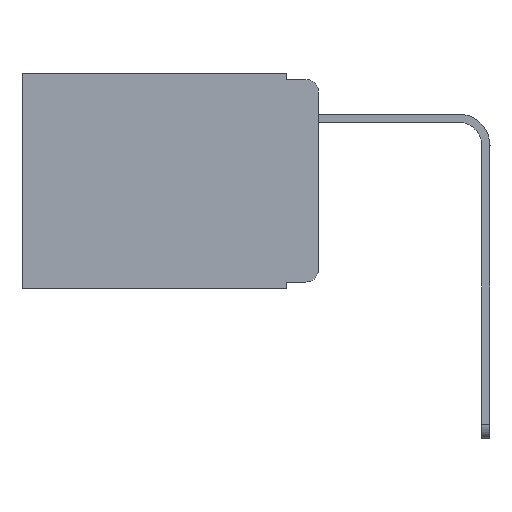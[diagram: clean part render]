
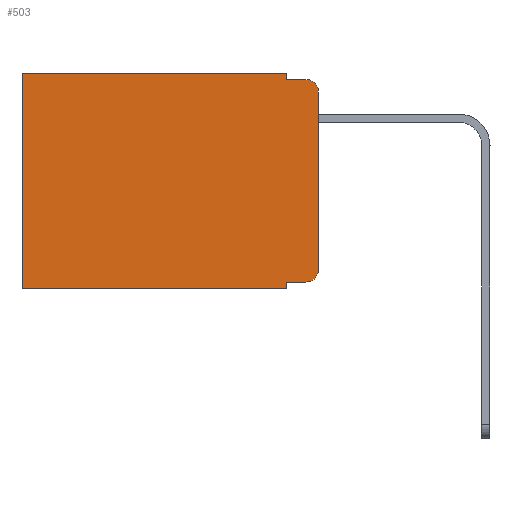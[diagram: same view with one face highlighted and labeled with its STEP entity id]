
A CAD part, left-side view. The second image highlights one B-rep face of the part: STEP entity #503.
In plain terms, the highlighted planar face has unit normal (-1, 0, 0).
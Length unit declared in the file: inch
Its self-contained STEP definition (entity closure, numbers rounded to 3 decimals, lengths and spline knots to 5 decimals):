
#73 = DIRECTION ( 'NONE',  ( 0., 0., -1. ) ) ;
#333 = EDGE_CURVE ( 'NONE', #14521, #5558, #12434, .T. ) ;
#384 = CARTESIAN_POINT ( 'NONE',  ( 0.298, 0., -0.313 ) ) ;
#451 = VECTOR ( 'NONE', #13434, 39.37008 ) ;
#503 = ADVANCED_FACE ( 'NONE', ( #1913 ), #4002, .F. ) ;
#621 = CARTESIAN_POINT ( 'NONE',  ( 0.298, 0.051, -0.333 ) ) ;
#686 = ORIENTED_EDGE ( 'NONE', *, *, #9910, .F. ) ;
#698 = CARTESIAN_POINT ( 'NONE',  ( 0.298, 0., -0.343 ) ) ;
#1372 = DIRECTION ( 'NONE',  ( 1., 0., 0. ) ) ;
#1875 = ORIENTED_EDGE ( 'NONE', *, *, #6727, .T. ) ;
#1913 = FACE_OUTER_BOUND ( 'NONE', #10948, .T. ) ;
#1921 = DIRECTION ( 'NONE',  ( 0., 1., 0. ) ) ;
#2101 = CARTESIAN_POINT ( 'NONE',  ( 0.298, 0.051, -0.01 ) ) ;
#2221 = ORIENTED_EDGE ( 'NONE', *, *, #333, .T. ) ;
#2616 = ORIENTED_EDGE ( 'NONE', *, *, #7275, .T. ) ;
#2718 = CARTESIAN_POINT ( 'NONE',  ( 0.298, 0.051, 0. ) ) ;
#2979 = VERTEX_POINT ( 'NONE', #384 ) ;
#3415 = DIRECTION ( 'NONE',  ( 0., -1., 0. ) ) ;
#3781 = LINE ( 'NONE', #2101, #11032 ) ;
#3963 = CARTESIAN_POINT ( 'NONE',  ( 0.298, 0.02, -0.01 ) ) ;
#3982 = VERTEX_POINT ( 'NONE', #7241 ) ;
#4002 = PLANE ( 'NONE',  #15668 ) ;
#4197 = ORIENTED_EDGE ( 'NONE', *, *, #6218, .F. ) ;
#4440 = VECTOR ( 'NONE', #14231, 39.37008 ) ;
#5270 = VERTEX_POINT ( 'NONE', #8256 ) ;
#5558 = VERTEX_POINT ( 'NONE', #6510 ) ;
#5615 = EDGE_CURVE ( 'NONE', #3982, #16295, #8392, .T. ) ;
#5673 = DIRECTION ( 'NONE',  ( 0., -1., 0. ) ) ;
#6050 = LINE ( 'NONE', #2718, #4440 ) ;
#6218 = EDGE_CURVE ( 'NONE', #5270, #12896, #6050, .T. ) ;
#6265 = AXIS2_PLACEMENT_3D ( 'NONE', #9762, #12261, #13597 ) ;
#6510 = CARTESIAN_POINT ( 'NONE',  ( 0.298, 0.02, -0.333 ) ) ;
#6727 = EDGE_CURVE ( 'NONE', #5558, #2979, #11082, .T. ) ;
#6936 = VERTEX_POINT ( 'NONE', #3963 ) ;
#7241 = CARTESIAN_POINT ( 'NONE',  ( 0.298, 0.473, 0. ) ) ;
#7275 = EDGE_CURVE ( 'NONE', #5270, #3982, #9014, .T. ) ;
#7451 = CARTESIAN_POINT ( 'NONE',  ( 0.298, 0.051, 0. ) ) ;
#7570 = VERTEX_POINT ( 'NONE', #10634 ) ;
#8256 = CARTESIAN_POINT ( 'NONE',  ( 0.298, 0.051, 0. ) ) ;
#8392 = LINE ( 'NONE', #15613, #14256 ) ;
#9014 = LINE ( 'NONE', #12173, #12670 ) ;
#9067 = EDGE_CURVE ( 'NONE', #14521, #7570, #15021, .T. ) ;
#9593 = VECTOR ( 'NONE', #5673, 39.37008 ) ;
#9727 = DIRECTION ( 'NONE',  ( 0., 1., 0. ) ) ;
#9762 = CARTESIAN_POINT ( 'NONE',  ( 0.298, 0.02, -0.03 ) ) ;
#9910 = EDGE_CURVE ( 'NONE', #12106, #2979, #11366, .T. ) ;
#10248 = DIRECTION ( 'NONE',  ( 0., 0., -1. ) ) ;
#10318 = ORIENTED_EDGE ( 'NONE', *, *, #12023, .F. ) ;
#10601 = EDGE_CURVE ( 'NONE', #12106, #6936, #16625, .T. ) ;
#10634 = CARTESIAN_POINT ( 'NONE',  ( 0.298, 0.051, -0.343 ) ) ;
#10767 = AXIS2_PLACEMENT_3D ( 'NONE', #15384, #15444, #16646 ) ;
#10898 = VECTOR ( 'NONE', #9727, 39.37008 ) ;
#10948 = EDGE_LOOP ( 'NONE', ( #686, #13343, #10318, #4197, #2616, #12401, #15115, #12839, #2221, #1875 ) ) ;
#11032 = VECTOR ( 'NONE', #3415, 39.37008 ) ;
#11082 = CIRCLE ( 'NONE', #10767, 0.02 ) ;
#11366 = LINE ( 'NONE', #13551, #451 ) ;
#11737 = DIRECTION ( 'NONE',  ( 0., 0., -1. ) ) ;
#12023 = EDGE_CURVE ( 'NONE', #12896, #6936, #3781, .T. ) ;
#12106 = VERTEX_POINT ( 'NONE', #14375 ) ;
#12173 = CARTESIAN_POINT ( 'NONE',  ( 0.298, 0., 0. ) ) ;
#12261 = DIRECTION ( 'NONE',  ( -1., 0., 0. ) ) ;
#12401 = ORIENTED_EDGE ( 'NONE', *, *, #5615, .T. ) ;
#12434 = LINE ( 'NONE', #621, #9593 ) ;
#12670 = VECTOR ( 'NONE', #1921, 39.37008 ) ;
#12839 = ORIENTED_EDGE ( 'NONE', *, *, #9067, .F. ) ;
#12896 = VERTEX_POINT ( 'NONE', #15937 ) ;
#13202 = EDGE_CURVE ( 'NONE', #7570, #16295, #16562, .T. ) ;
#13343 = ORIENTED_EDGE ( 'NONE', *, *, #10601, .T. ) ;
#13434 = DIRECTION ( 'NONE',  ( 0., 0., -1. ) ) ;
#13551 = CARTESIAN_POINT ( 'NONE',  ( 0.298, 0., 0. ) ) ;
#13597 = DIRECTION ( 'NONE',  ( 0., 0., -1. ) ) ;
#14088 = CARTESIAN_POINT ( 'NONE',  ( 0.298, 0., 0. ) ) ;
#14228 = CARTESIAN_POINT ( 'NONE',  ( 0.298, 0.051, -0.333 ) ) ;
#14231 = DIRECTION ( 'NONE',  ( 0., 0., -1. ) ) ;
#14256 = VECTOR ( 'NONE', #10248, 39.37008 ) ;
#14375 = CARTESIAN_POINT ( 'NONE',  ( 0.298, 0., -0.03 ) ) ;
#14521 = VERTEX_POINT ( 'NONE', #14228 ) ;
#14604 = VECTOR ( 'NONE', #73, 39.37008 ) ;
#15021 = LINE ( 'NONE', #7451, #14604 ) ;
#15115 = ORIENTED_EDGE ( 'NONE', *, *, #13202, .F. ) ;
#15384 = CARTESIAN_POINT ( 'NONE',  ( 0.298, 0.02, -0.313 ) ) ;
#15444 = DIRECTION ( 'NONE',  ( -1., 0., 0. ) ) ;
#15599 = CARTESIAN_POINT ( 'NONE',  ( 0.298, 0.473, -0.343 ) ) ;
#15613 = CARTESIAN_POINT ( 'NONE',  ( 0.298, 0.473, 0. ) ) ;
#15668 = AXIS2_PLACEMENT_3D ( 'NONE', #14088, #1372, #11737 ) ;
#15937 = CARTESIAN_POINT ( 'NONE',  ( 0.298, 0.051, -0.01 ) ) ;
#16295 = VERTEX_POINT ( 'NONE', #15599 ) ;
#16562 = LINE ( 'NONE', #698, #10898 ) ;
#16625 = CIRCLE ( 'NONE', #6265, 0.02 ) ;
#16646 = DIRECTION ( 'NONE',  ( 0., 0., -1. ) ) ;
